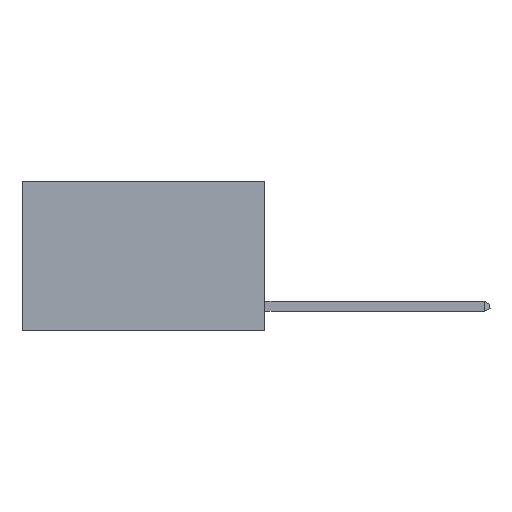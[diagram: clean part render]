
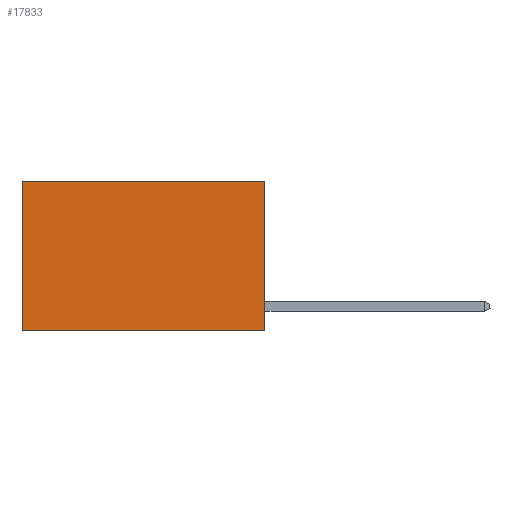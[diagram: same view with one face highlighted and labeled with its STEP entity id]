
A CAD part, left-side view. The second image highlights one B-rep face of the part: STEP entity #17833.
In plain terms, the highlighted planar face has unit normal (-1, 0, 0).
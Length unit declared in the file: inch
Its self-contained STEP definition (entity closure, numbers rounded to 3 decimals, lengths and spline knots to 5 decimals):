
#1066 = AXIS2_PLACEMENT_3D ( 'NONE', #6903, #3263, #18489 ) ;
#1220 = LINE ( 'NONE', #14237, #5262 ) ;
#2142 = DIRECTION ( 'NONE',  ( 0., 0., -1. ) ) ;
#3263 = DIRECTION ( 'NONE',  ( 1., 0., 0. ) ) ;
#3482 = DIRECTION ( 'NONE',  ( 0., 0., -1. ) ) ;
#5068 = LINE ( 'NONE', #19968, #15037 ) ;
#5145 = CARTESIAN_POINT ( 'NONE',  ( 0.2625, 0.6, 0. ) ) ;
#5262 = VECTOR ( 'NONE', #2142, 39.37008 ) ;
#5844 = CARTESIAN_POINT ( 'NONE',  ( 0.2625, 0.6, -0.37 ) ) ;
#6303 = DIRECTION ( 'NONE',  ( 0., 1., 0. ) ) ;
#6794 = VERTEX_POINT ( 'NONE', #17278 ) ;
#6903 = CARTESIAN_POINT ( 'NONE',  ( 0.2625, 0., 0. ) ) ;
#7020 = VECTOR ( 'NONE', #3482, 39.37008 ) ;
#8353 = FACE_OUTER_BOUND ( 'NONE', #20023, .T. ) ;
#8834 = ORIENTED_EDGE ( 'NONE', *, *, #10000, .F. ) ;
#9818 = VERTEX_POINT ( 'NONE', #18969 ) ;
#10000 = EDGE_CURVE ( 'NONE', #9818, #12664, #5068, .T. ) ;
#10030 = CARTESIAN_POINT ( 'NONE',  ( 0.2625, 0., 0. ) ) ;
#10329 = PLANE ( 'NONE',  #1066 ) ;
#12664 = VERTEX_POINT ( 'NONE', #5844 ) ;
#12848 = CARTESIAN_POINT ( 'NONE',  ( 0.2625, 0., 0. ) ) ;
#14237 = CARTESIAN_POINT ( 'NONE',  ( 0.2625, 0., 0. ) ) ;
#14775 = EDGE_CURVE ( 'NONE', #18439, #9818, #1220, .T. ) ;
#15037 = VECTOR ( 'NONE', #6303, 39.37008 ) ;
#15568 = ORIENTED_EDGE ( 'NONE', *, *, #16090, .T. ) ;
#15764 = ORIENTED_EDGE ( 'NONE', *, *, #14775, .F. ) ;
#16090 = EDGE_CURVE ( 'NONE', #6794, #12664, #20359, .T. ) ;
#16828 = DIRECTION ( 'NONE',  ( 0., 1., 0. ) ) ;
#17278 = CARTESIAN_POINT ( 'NONE',  ( 0.2625, 0.6, 0. ) ) ;
#17833 = ADVANCED_FACE ( 'NONE', ( #8353 ), #10329, .F. ) ;
#18439 = VERTEX_POINT ( 'NONE', #12848 ) ;
#18481 = VECTOR ( 'NONE', #16828, 39.37008 ) ;
#18489 = DIRECTION ( 'NONE',  ( 0., 0., -1. ) ) ;
#18586 = EDGE_CURVE ( 'NONE', #18439, #6794, #20168, .T. ) ;
#18969 = CARTESIAN_POINT ( 'NONE',  ( 0.2625, 0., -0.37 ) ) ;
#19968 = CARTESIAN_POINT ( 'NONE',  ( 0.2625, 0., -0.37 ) ) ;
#20023 = EDGE_LOOP ( 'NONE', ( #15568, #8834, #15764, #21093 ) ) ;
#20168 = LINE ( 'NONE', #10030, #18481 ) ;
#20359 = LINE ( 'NONE', #5145, #7020 ) ;
#21093 = ORIENTED_EDGE ( 'NONE', *, *, #18586, .T. ) ;
